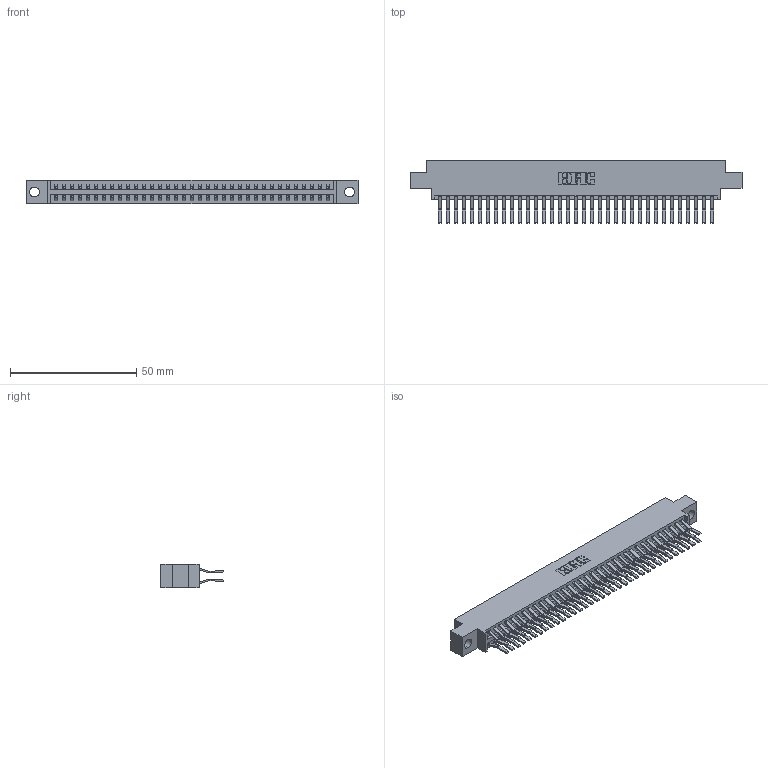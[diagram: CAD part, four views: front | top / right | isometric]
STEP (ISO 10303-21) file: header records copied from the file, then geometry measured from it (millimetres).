
FILE_DESCRIPTION (( 'STEP AP203' ), '1' );
FILE_NAME ('346-070-560-804.STEP', '2022-05-24T22:46:20', ( '' ), ( '' ), 'SwSTEP 2.0', 'SolidWorks 2020', '' );
FILE_SCHEMA (( 'CONFIG_CONTROL_DESIGN' ));
Length unit declared in the file: inch
Products named in the file (3): 346-070-560-804; 345-292-001_560 Tail; 346 Part_0.170 Offset - 0.156 Dia-TH
Assembly tree (71 placements, depth 2):
  346-070-560-804
    346 Part_0.170 Offset - 0.156 Dia-TH
    345-292-001_560 Tail  x70
Bounding box: 131.7 x 24.78 x 9.4 mm (x, y, z)
Volume: 12986.2 mm3; surface area: 18992 mm2
Topology: 71 solids, 71 shells, 3920 faces, 11647 edges, 7670 vertices
Faces by surface type: plane 2544, cylinder 1376
Entity records: 24423 total; most frequent: CARTESIAN_POINT 4042, ORIENTED_EDGE 3974, DIRECTION 3615, EDGE_CURVE 1987, VECTOR 1711, LINE 1711, VERTEX_POINT 1322, AXIS2_PLACEMENT_3D 952
